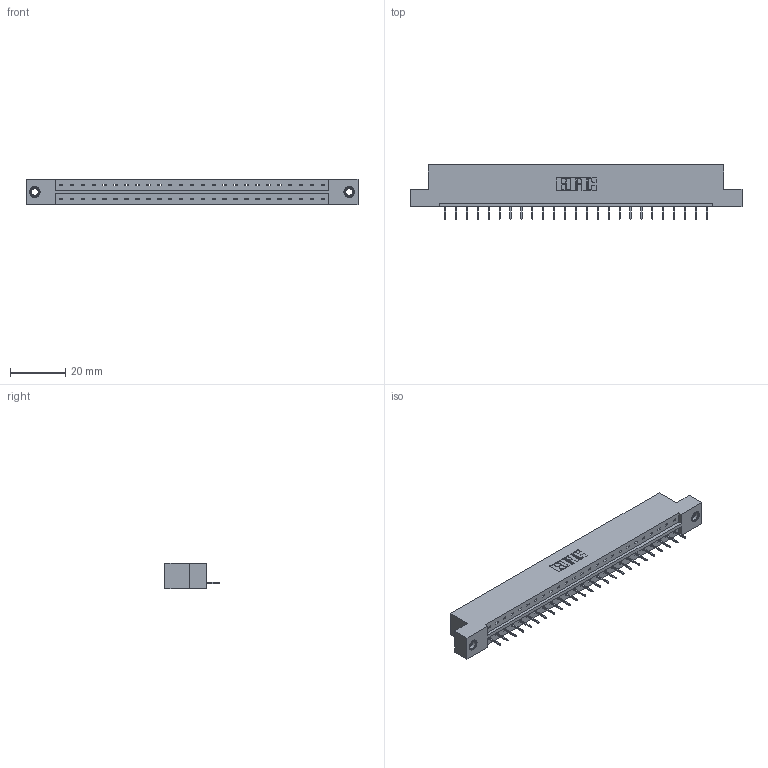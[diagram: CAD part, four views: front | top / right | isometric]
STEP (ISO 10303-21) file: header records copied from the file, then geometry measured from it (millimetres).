
FILE_DESCRIPTION (( 'STEP AP203' ), '1' );
FILE_NAME ('333-025-524-107.STEP', '2018-08-02T12:03:33', ( '' ), ( '' ), 'SwSTEP 2.0', 'SolidWorks 2016', '' );
FILE_SCHEMA (( 'CONFIG_CONTROL_DESIGN' ));
Length unit declared in the file: inch
Products named in the file (4): 345-292-001_345-293-124; 345-250-001_345-250-005-103; 333-025-524-107; 333 Part_Flush - .156 Dia - TI
Assembly tree (28 placements, depth 2):
  333-025-524-107
    333 Part_Flush - .156 Dia - TI
    345-292-001_345-293-124  x25
    345-250-001_345-250-005-103  x2
Bounding box: 120.6 x 19.69 x 9.4 mm (x, y, z)
Volume: 11877.2 mm3; surface area: 12437.8 mm2
Topology: 28 solids, 28 shells, 1724 faces, 4947 edges, 3190 vertices
Faces by surface type: plane 1302, cylinder 406, cone 12, torus 4
Entity records: 18742 total; most frequent: CARTESIAN_POINT 3216, ORIENTED_EDGE 3170, DIRECTION 2781, EDGE_CURVE 1585, LINE 1441, VECTOR 1441, VERTEX_POINT 1048, AXIS2_PLACEMENT_3D 670
